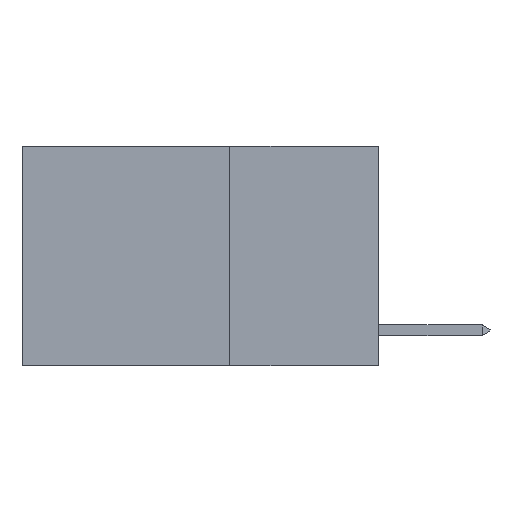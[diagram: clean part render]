
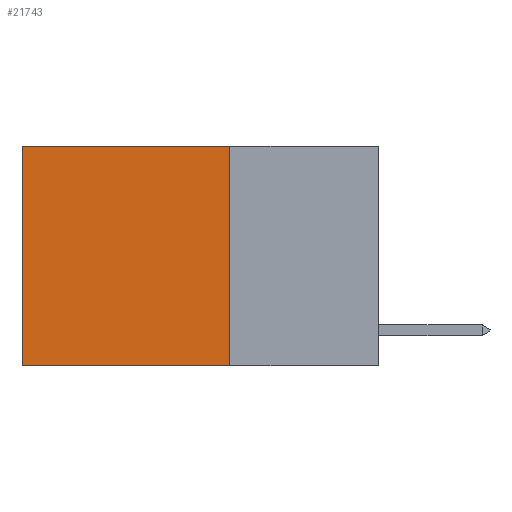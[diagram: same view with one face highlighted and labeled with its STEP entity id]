
A CAD part, left-side view. The second image highlights one B-rep face of the part: STEP entity #21743.
In plain terms, the highlighted planar face has unit normal (-1, 0, 0).
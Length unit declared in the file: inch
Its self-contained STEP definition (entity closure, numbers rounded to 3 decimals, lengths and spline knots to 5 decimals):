
#694 = LINE ( 'NONE', #7210, #12240 ) ;
#925 = EDGE_LOOP ( 'NONE', ( #29783, #7037, #3555, #28881 ) ) ;
#1749 = LINE ( 'NONE', #27781, #7185 ) ;
#2363 = DIRECTION ( 'NONE',  ( 0., 0., -1. ) ) ;
#2708 = DIRECTION ( 'NONE',  ( 0., 0., -1. ) ) ;
#3002 = CARTESIAN_POINT ( 'NONE',  ( 0.2625, 0.25, -0.37 ) ) ;
#3289 = VERTEX_POINT ( 'NONE', #3002 ) ;
#3555 = ORIENTED_EDGE ( 'NONE', *, *, #11832, .F. ) ;
#5209 = LINE ( 'NONE', #25953, #28449 ) ;
#5995 = DIRECTION ( 'NONE',  ( 1., 0., 0. ) ) ;
#6957 = DIRECTION ( 'NONE',  ( 0., 1., 0. ) ) ;
#7037 = ORIENTED_EDGE ( 'NONE', *, *, #17537, .F. ) ;
#7185 = VECTOR ( 'NONE', #6957, 39.37008 ) ;
#7210 = CARTESIAN_POINT ( 'NONE',  ( 0.2625, 0.25, 0. ) ) ;
#7812 = CARTESIAN_POINT ( 'NONE',  ( 0.2625, 0.6, -0.37 ) ) ;
#8201 = CARTESIAN_POINT ( 'NONE',  ( 0.2625, 0.25, 0. ) ) ;
#8311 = VERTEX_POINT ( 'NONE', #7812 ) ;
#8973 = VECTOR ( 'NONE', #2363, 39.37008 ) ;
#10213 = AXIS2_PLACEMENT_3D ( 'NONE', #8201, #5995, #22236 ) ;
#11832 = EDGE_CURVE ( 'NONE', #13373, #3289, #5209, .T. ) ;
#12240 = VECTOR ( 'NONE', #25798, 39.37008 ) ;
#13196 = CARTESIAN_POINT ( 'NONE',  ( 0.2625, 0.25, 0. ) ) ;
#13373 = VERTEX_POINT ( 'NONE', #13196 ) ;
#14259 = EDGE_CURVE ( 'NONE', #14629, #8311, #21381, .T. ) ;
#14629 = VERTEX_POINT ( 'NONE', #19881 ) ;
#17537 = EDGE_CURVE ( 'NONE', #3289, #8311, #1749, .T. ) ;
#19881 = CARTESIAN_POINT ( 'NONE',  ( 0.2625, 0.6, 0. ) ) ;
#19888 = PLANE ( 'NONE',  #10213 ) ;
#20925 = CARTESIAN_POINT ( 'NONE',  ( 0.2625, 0.6, 0. ) ) ;
#21381 = LINE ( 'NONE', #20925, #8973 ) ;
#21743 = ADVANCED_FACE ( 'NONE', ( #22933 ), #19888, .F. ) ;
#22236 = DIRECTION ( 'NONE',  ( 0., 0., -1. ) ) ;
#22933 = FACE_OUTER_BOUND ( 'NONE', #925, .T. ) ;
#25798 = DIRECTION ( 'NONE',  ( 0., 1., 0. ) ) ;
#25953 = CARTESIAN_POINT ( 'NONE',  ( 0.2625, 0.25, 0. ) ) ;
#27781 = CARTESIAN_POINT ( 'NONE',  ( 0.2625, 0.25, -0.37 ) ) ;
#28449 = VECTOR ( 'NONE', #2708, 39.37008 ) ;
#28881 = ORIENTED_EDGE ( 'NONE', *, *, #29026, .T. ) ;
#29026 = EDGE_CURVE ( 'NONE', #13373, #14629, #694, .T. ) ;
#29783 = ORIENTED_EDGE ( 'NONE', *, *, #14259, .T. ) ;
